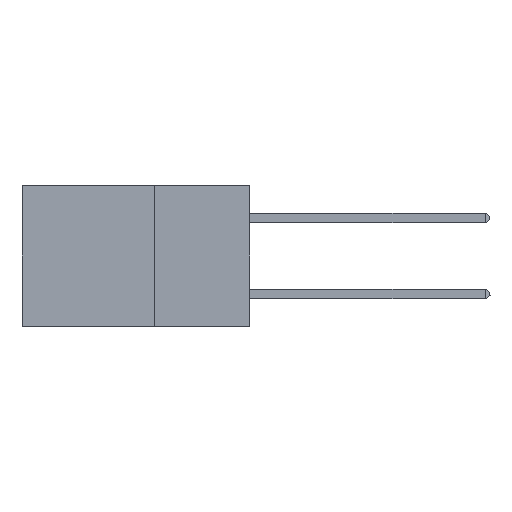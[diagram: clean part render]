
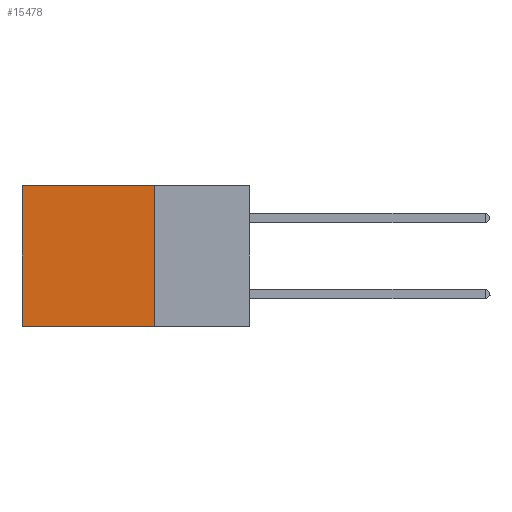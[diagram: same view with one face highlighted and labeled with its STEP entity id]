
A CAD part, left-side view. The second image highlights one B-rep face of the part: STEP entity #15478.
In plain terms, the highlighted planar face has unit normal (-1, 0, 0).
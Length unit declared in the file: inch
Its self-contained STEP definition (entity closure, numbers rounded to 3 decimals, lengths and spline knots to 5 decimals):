
#1985 = CARTESIAN_POINT ( 'NONE',  ( 0.2875, 0.25, 0. ) ) ;
#2758 = LINE ( 'NONE', #39374, #20937 ) ;
#3373 = ORIENTED_EDGE ( 'NONE', *, *, #32780, .T. ) ;
#4095 = ORIENTED_EDGE ( 'NONE', *, *, #36169, .T. ) ;
#5046 = VERTEX_POINT ( 'NONE', #31195 ) ;
#5122 = FACE_OUTER_BOUND ( 'NONE', #19784, .T. ) ;
#7964 = DIRECTION ( 'NONE',  ( 0., 1., 0. ) ) ;
#8856 = LINE ( 'NONE', #23183, #10777 ) ;
#9873 = CARTESIAN_POINT ( 'NONE',  ( 0.2875, 0.6, -0.37 ) ) ;
#9981 = ORIENTED_EDGE ( 'NONE', *, *, #11035, .F. ) ;
#10777 = VECTOR ( 'NONE', #7964, 39.37008 ) ;
#11035 = EDGE_CURVE ( 'NONE', #5046, #38770, #8856, .T. ) ;
#11204 = ORIENTED_EDGE ( 'NONE', *, *, #14105, .F. ) ;
#11349 = AXIS2_PLACEMENT_3D ( 'NONE', #35587, #17363, #32114 ) ;
#11998 = VECTOR ( 'NONE', #37502, 39.37008 ) ;
#12901 = VECTOR ( 'NONE', #17372, 39.37008 ) ;
#14010 = PLANE ( 'NONE',  #11349 ) ;
#14105 = EDGE_CURVE ( 'NONE', #23226, #5046, #38687, .T. ) ;
#14345 = CARTESIAN_POINT ( 'NONE',  ( 0.2875, 0.6, 0. ) ) ;
#15478 = ADVANCED_FACE ( 'NONE', ( #5122 ), #14010, .F. ) ;
#17363 = DIRECTION ( 'NONE',  ( 1., 0., 0. ) ) ;
#17372 = DIRECTION ( 'NONE',  ( 0., 0., -1. ) ) ;
#17474 = CARTESIAN_POINT ( 'NONE',  ( 0.2875, 0.25, 0. ) ) ;
#19784 = EDGE_LOOP ( 'NONE', ( #4095, #9981, #11204, #3373 ) ) ;
#20937 = VECTOR ( 'NONE', #27632, 39.37008 ) ;
#22690 = CARTESIAN_POINT ( 'NONE',  ( 0.2875, 0.25, 0. ) ) ;
#23183 = CARTESIAN_POINT ( 'NONE',  ( 0.2875, 0.25, -0.37 ) ) ;
#23226 = VERTEX_POINT ( 'NONE', #17474 ) ;
#27632 = DIRECTION ( 'NONE',  ( 0., 0., -1. ) ) ;
#27772 = LINE ( 'NONE', #22690, #11998 ) ;
#31195 = CARTESIAN_POINT ( 'NONE',  ( 0.2875, 0.25, -0.37 ) ) ;
#32114 = DIRECTION ( 'NONE',  ( 0., 0., -1. ) ) ;
#32780 = EDGE_CURVE ( 'NONE', #23226, #35844, #27772, .T. ) ;
#35587 = CARTESIAN_POINT ( 'NONE',  ( 0.2875, 0.25, 0. ) ) ;
#35844 = VERTEX_POINT ( 'NONE', #14345 ) ;
#36169 = EDGE_CURVE ( 'NONE', #35844, #38770, #2758, .T. ) ;
#37502 = DIRECTION ( 'NONE',  ( 0., 1., 0. ) ) ;
#38687 = LINE ( 'NONE', #1985, #12901 ) ;
#38770 = VERTEX_POINT ( 'NONE', #9873 ) ;
#39374 = CARTESIAN_POINT ( 'NONE',  ( 0.2875, 0.6, 0. ) ) ;
